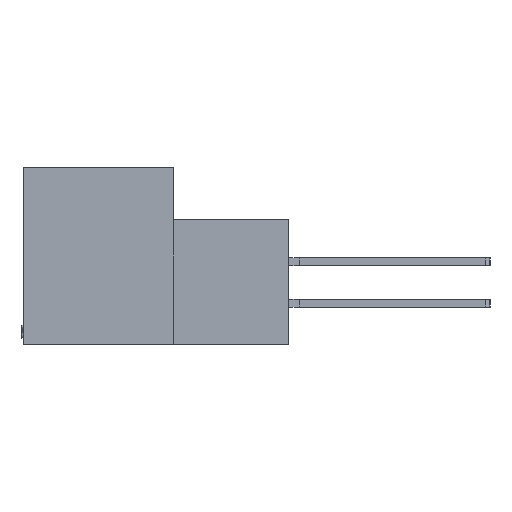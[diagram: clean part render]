
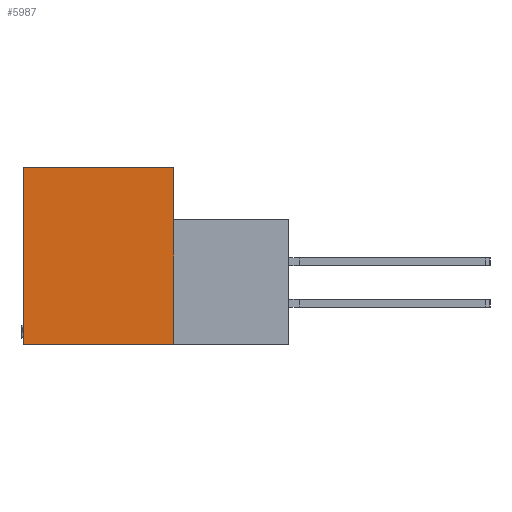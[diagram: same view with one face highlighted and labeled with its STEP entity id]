
A CAD part, left-side view. The second image highlights one B-rep face of the part: STEP entity #5987.
In plain terms, the highlighted planar face has unit normal (-1, 0, 0).
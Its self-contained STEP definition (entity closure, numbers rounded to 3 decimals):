
#2016 = ORIENTED_EDGE ( 'NONE', *, *, #31137, .F. ) ;
#3082 = CARTESIAN_POINT ( 'NONE',  ( 0., 0., 0. ) ) ;
#3373 = DIRECTION ( 'NONE',  ( 0., 1., 0. ) ) ;
#3703 = LINE ( 'NONE', #3082, #42360 ) ;
#5229 = VERTEX_POINT ( 'NONE', #9070 ) ;
#5987 = ADVANCED_FACE ( 'NONE', ( #19919 ), #25468, .F. ) ;
#6274 = VERTEX_POINT ( 'NONE', #37294 ) ;
#8486 = DIRECTION ( 'NONE',  ( 0., 0., 1. ) ) ;
#9070 = CARTESIAN_POINT ( 'NONE',  ( 0., 11.506, 0. ) ) ;
#9434 = ORIENTED_EDGE ( 'NONE', *, *, #32182, .F. ) ;
#9950 = LINE ( 'NONE', #17860, #38607 ) ;
#10291 = DIRECTION ( 'NONE',  ( 0., -1., 0. ) ) ;
#12320 = CARTESIAN_POINT ( 'NONE',  ( 0., 11.506, -13.487 ) ) ;
#16502 = EDGE_CURVE ( 'NONE', #21893, #6274, #9950, .T. ) ;
#17860 = CARTESIAN_POINT ( 'NONE',  ( 0., -8.814, -13.487 ) ) ;
#19919 = FACE_OUTER_BOUND ( 'NONE', #34486, .T. ) ;
#20781 = VECTOR ( 'NONE', #8486, 1000. ) ;
#21592 = DIRECTION ( 'NONE',  ( 0., 0., -1. ) ) ;
#21858 = LINE ( 'NONE', #12320, #20781 ) ;
#21893 = VERTEX_POINT ( 'NONE', #35511 ) ;
#24261 = EDGE_CURVE ( 'NONE', #5229, #26689, #37353, .T. ) ;
#25468 = PLANE ( 'NONE',  #28407 ) ;
#26689 = VERTEX_POINT ( 'NONE', #33027 ) ;
#27870 = CARTESIAN_POINT ( 'NONE',  ( 0., 11.506, 0. ) ) ;
#28407 = AXIS2_PLACEMENT_3D ( 'NONE', #32374, #28824, #21592 ) ;
#28539 = VECTOR ( 'NONE', #10291, 1000. ) ;
#28824 = DIRECTION ( 'NONE',  ( 1., 0., 0. ) ) ;
#31137 = EDGE_CURVE ( 'NONE', #26689, #21893, #3703, .T. ) ;
#32182 = EDGE_CURVE ( 'NONE', #6274, #5229, #21858, .T. ) ;
#32374 = CARTESIAN_POINT ( 'NONE',  ( 0., 0., 0. ) ) ;
#33027 = CARTESIAN_POINT ( 'NONE',  ( 0., 0., 0. ) ) ;
#33398 = ORIENTED_EDGE ( 'NONE', *, *, #16502, .F. ) ;
#34140 = ORIENTED_EDGE ( 'NONE', *, *, #24261, .F. ) ;
#34486 = EDGE_LOOP ( 'NONE', ( #33398, #2016, #34140, #9434 ) ) ;
#35511 = CARTESIAN_POINT ( 'NONE',  ( 0., 0., -13.487 ) ) ;
#37294 = CARTESIAN_POINT ( 'NONE',  ( 0., 11.506, -13.487 ) ) ;
#37353 = LINE ( 'NONE', #27870, #28539 ) ;
#38607 = VECTOR ( 'NONE', #3373, 1000. ) ;
#42360 = VECTOR ( 'NONE', #45522, 1000. ) ;
#45522 = DIRECTION ( 'NONE',  ( 0., 0., -1. ) ) ;
